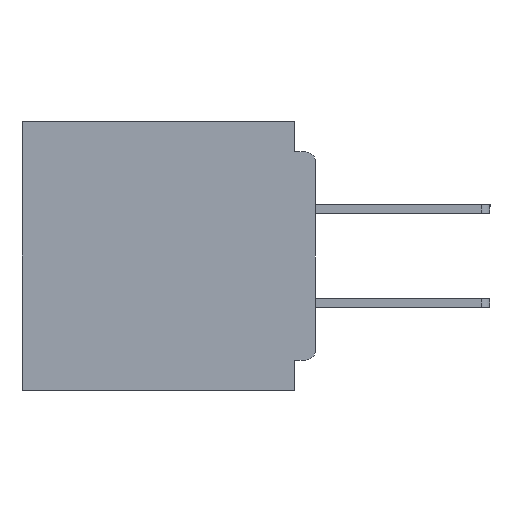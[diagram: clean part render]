
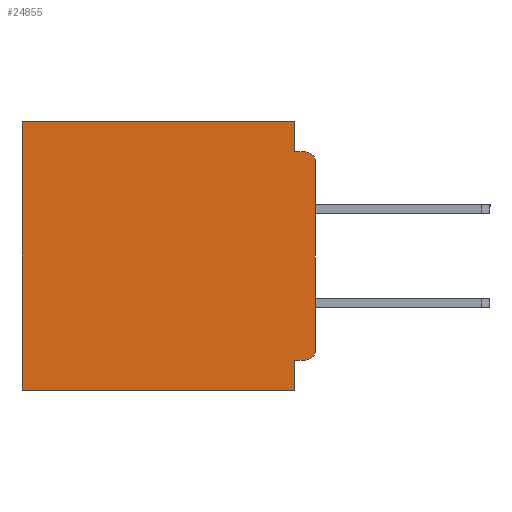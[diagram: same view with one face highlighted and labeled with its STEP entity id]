
A CAD part, left-side view. The second image highlights one B-rep face of the part: STEP entity #24855.
In plain terms, the highlighted planar face has unit normal (-1, 0, 0).
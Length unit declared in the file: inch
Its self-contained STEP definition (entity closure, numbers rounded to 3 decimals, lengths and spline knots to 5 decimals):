
#701 = CARTESIAN_POINT ( 'NONE',  ( 0.3, 0.031, -0.045 ) ) ;
#1168 = VECTOR ( 'NONE', #3033, 39.37008 ) ;
#1342 = ORIENTED_EDGE ( 'NONE', *, *, #31049, .F. ) ;
#1349 = EDGE_CURVE ( 'NONE', #4096, #18045, #32238, .T. ) ;
#1885 = LINE ( 'NONE', #31107, #31140 ) ;
#2705 = VERTEX_POINT ( 'NONE', #22883 ) ;
#2775 = CARTESIAN_POINT ( 'NONE',  ( 0.3, 0.031, 0. ) ) ;
#2971 = VERTEX_POINT ( 'NONE', #16418 ) ;
#3008 = DIRECTION ( 'NONE',  ( 0., 0., -1. ) ) ;
#3033 = DIRECTION ( 'NONE',  ( 0., 0., -1. ) ) ;
#3508 = CARTESIAN_POINT ( 'NONE',  ( 0.3, 0., -0.355 ) ) ;
#4048 = EDGE_CURVE ( 'NONE', #25310, #2705, #36401, .T. ) ;
#4096 = VERTEX_POINT ( 'NONE', #11216 ) ;
#4205 = CARTESIAN_POINT ( 'NONE',  ( 0.3, 0., -0.045 ) ) ;
#4247 = DIRECTION ( 'NONE',  ( -1., 0., 0. ) ) ;
#4694 = VECTOR ( 'NONE', #33535, 39.37008 ) ;
#5053 = DIRECTION ( 'NONE',  ( -1., 0., 0. ) ) ;
#5133 = CARTESIAN_POINT ( 'NONE',  ( 0.3, 0.015, -0.06 ) ) ;
#5189 = CARTESIAN_POINT ( 'NONE',  ( 0.3, 0.437, 0. ) ) ;
#5228 = CARTESIAN_POINT ( 'NONE',  ( 0.3, 0.015, -0.045 ) ) ;
#5452 = VERTEX_POINT ( 'NONE', #35917 ) ;
#5629 = EDGE_CURVE ( 'NONE', #2971, #13668, #16874, .T. ) ;
#7206 = DIRECTION ( 'NONE',  ( 0., -1., 0. ) ) ;
#8174 = EDGE_CURVE ( 'NONE', #2705, #13025, #32447, .T. ) ;
#10304 = CARTESIAN_POINT ( 'NONE',  ( 0.3, 0.437, -0.4 ) ) ;
#10506 = ORIENTED_EDGE ( 'NONE', *, *, #5629, .T. ) ;
#11216 = CARTESIAN_POINT ( 'NONE',  ( 0.3, 0.031, 0. ) ) ;
#11482 = EDGE_LOOP ( 'NONE', ( #1342, #10506, #30393, #36978, #32613, #17251, #30830, #12721, #16781, #19266 ) ) ;
#11881 = AXIS2_PLACEMENT_3D ( 'NONE', #5133, #5053, #3008 ) ;
#12721 = ORIENTED_EDGE ( 'NONE', *, *, #8174, .F. ) ;
#12757 = VECTOR ( 'NONE', #16342, 39.37008 ) ;
#12983 = VECTOR ( 'NONE', #28311, 39.37008 ) ;
#13025 = VERTEX_POINT ( 'NONE', #36601 ) ;
#13668 = VERTEX_POINT ( 'NONE', #5228 ) ;
#14449 = VECTOR ( 'NONE', #34705, 39.37008 ) ;
#16060 = CIRCLE ( 'NONE', #24401, 0.015 ) ;
#16253 = PLANE ( 'NONE',  #17509 ) ;
#16342 = DIRECTION ( 'NONE',  ( 0., 1., 0. ) ) ;
#16385 = DIRECTION ( 'NONE',  ( 0., 0., -1. ) ) ;
#16418 = CARTESIAN_POINT ( 'NONE',  ( 0.3, 0., -0.06 ) ) ;
#16459 = CARTESIAN_POINT ( 'NONE',  ( 0.3, 0.031, -0.4 ) ) ;
#16781 = ORIENTED_EDGE ( 'NONE', *, *, #4048, .F. ) ;
#16874 = CIRCLE ( 'NONE', #11881, 0.015 ) ;
#17251 = ORIENTED_EDGE ( 'NONE', *, *, #26226, .T. ) ;
#17509 = AXIS2_PLACEMENT_3D ( 'NONE', #25013, #33642, #16385 ) ;
#18045 = VERTEX_POINT ( 'NONE', #701 ) ;
#19137 = EDGE_CURVE ( 'NONE', #18045, #13668, #21650, .T. ) ;
#19266 = ORIENTED_EDGE ( 'NONE', *, *, #28407, .T. ) ;
#21650 = LINE ( 'NONE', #4205, #28370 ) ;
#21866 = CARTESIAN_POINT ( 'NONE',  ( 0.3, 0.015, -0.34 ) ) ;
#22193 = CARTESIAN_POINT ( 'NONE',  ( 0.3, 0.015, -0.355 ) ) ;
#22210 = LINE ( 'NONE', #26120, #14449 ) ;
#22560 = CARTESIAN_POINT ( 'NONE',  ( 0.3, 0., -0.4 ) ) ;
#22883 = CARTESIAN_POINT ( 'NONE',  ( 0.3, 0.031, -0.355 ) ) ;
#23066 = VERTEX_POINT ( 'NONE', #10304 ) ;
#24103 = FACE_OUTER_BOUND ( 'NONE', #11482, .T. ) ;
#24401 = AXIS2_PLACEMENT_3D ( 'NONE', #21866, #4247, #24740 ) ;
#24740 = DIRECTION ( 'NONE',  ( 0., 0., -1. ) ) ;
#24820 = VECTOR ( 'NONE', #36489, 39.37008 ) ;
#24855 = ADVANCED_FACE ( 'NONE', ( #24103 ), #16253, .F. ) ;
#25013 = CARTESIAN_POINT ( 'NONE',  ( 0.3, 0., -0.4 ) ) ;
#25310 = VERTEX_POINT ( 'NONE', #22193 ) ;
#26120 = CARTESIAN_POINT ( 'NONE',  ( 0.3, 0.437, -0.4 ) ) ;
#26226 = EDGE_CURVE ( 'NONE', #31735, #23066, #22210, .T. ) ;
#27346 = EDGE_CURVE ( 'NONE', #13025, #23066, #36773, .T. ) ;
#28311 = DIRECTION ( 'NONE',  ( 0., 1., 0. ) ) ;
#28370 = VECTOR ( 'NONE', #7206, 39.37008 ) ;
#28407 = EDGE_CURVE ( 'NONE', #25310, #5452, #16060, .T. ) ;
#30393 = ORIENTED_EDGE ( 'NONE', *, *, #19137, .F. ) ;
#30830 = ORIENTED_EDGE ( 'NONE', *, *, #27346, .F. ) ;
#31049 = EDGE_CURVE ( 'NONE', #2971, #5452, #1885, .T. ) ;
#31107 = CARTESIAN_POINT ( 'NONE',  ( 0.3, 0., -0.4 ) ) ;
#31140 = VECTOR ( 'NONE', #33942, 39.37008 ) ;
#31735 = VERTEX_POINT ( 'NONE', #5189 ) ;
#32238 = LINE ( 'NONE', #2775, #1168 ) ;
#32447 = LINE ( 'NONE', #16459, #24820 ) ;
#32613 = ORIENTED_EDGE ( 'NONE', *, *, #35966, .T. ) ;
#33535 = DIRECTION ( 'NONE',  ( 0., 1., 0. ) ) ;
#33642 = DIRECTION ( 'NONE',  ( 1., 0., 0. ) ) ;
#33942 = DIRECTION ( 'NONE',  ( 0., 0., -1. ) ) ;
#34705 = DIRECTION ( 'NONE',  ( 0., 0., -1. ) ) ;
#35672 = LINE ( 'NONE', #36391, #12757 ) ;
#35917 = CARTESIAN_POINT ( 'NONE',  ( 0.3, 0., -0.34 ) ) ;
#35966 = EDGE_CURVE ( 'NONE', #4096, #31735, #35672, .T. ) ;
#36391 = CARTESIAN_POINT ( 'NONE',  ( 0.3, 0., 0. ) ) ;
#36401 = LINE ( 'NONE', #3508, #4694 ) ;
#36489 = DIRECTION ( 'NONE',  ( 0., 0., -1. ) ) ;
#36601 = CARTESIAN_POINT ( 'NONE',  ( 0.3, 0.031, -0.4 ) ) ;
#36773 = LINE ( 'NONE', #22560, #12983 ) ;
#36978 = ORIENTED_EDGE ( 'NONE', *, *, #1349, .F. ) ;
